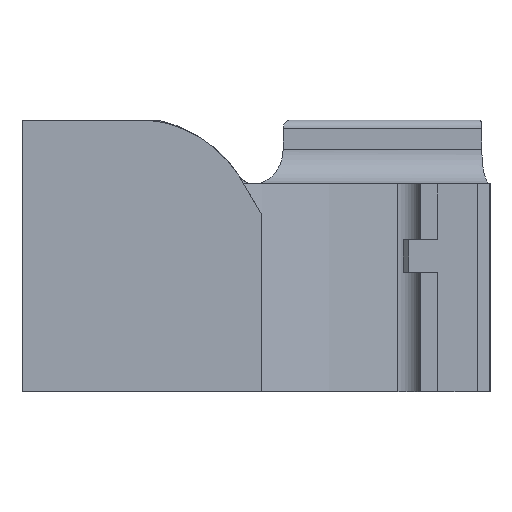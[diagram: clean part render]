
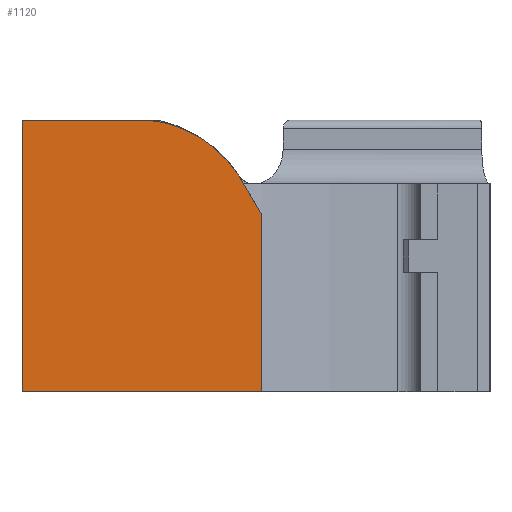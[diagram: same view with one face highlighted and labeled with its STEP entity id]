
A CAD part, front view. The second image highlights one B-rep face of the part: STEP entity #1120.
In plain terms, the highlighted planar face has unit normal (0, -1, 0).
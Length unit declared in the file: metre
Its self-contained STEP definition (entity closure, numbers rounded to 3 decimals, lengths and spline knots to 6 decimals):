
#39=PLANE('',#1247);
#86=FACE_OUTER_BOUND('',#145,.T.);
#145=EDGE_LOOP('',(#937,#938,#939,#940,#941,#942));
#189=LINE('',#1629,#303);
#198=LINE('',#1653,#312);
#215=LINE('',#1703,#329);
#235=LINE('',#1781,#349);
#240=LINE('',#1798,#354);
#303=VECTOR('',#1289,0.01);
#312=VECTOR('',#1310,0.01);
#329=VECTOR('',#1353,0.016179);
#349=VECTOR('',#1417,0.014606);
#354=VECTOR('',#1432,0.01);
#416=CIRCLE('',#1175,0.005582);
#457=VERTEX_POINT('',#1626);
#458=VERTEX_POINT('',#1628);
#460=VERTEX_POINT('',#1634);
#467=VERTEX_POINT('',#1652);
#487=VERTEX_POINT('',#1702);
#523=VERTEX_POINT('',#1779);
#568=EDGE_CURVE('',#458,#457,#189,.T.);
#572=EDGE_CURVE('',#457,#460,#416,.T.);
#580=EDGE_CURVE('',#467,#458,#198,.T.);
#605=EDGE_CURVE('',#487,#467,#215,.T.);
#645=EDGE_CURVE('',#523,#460,#235,.T.);
#652=EDGE_CURVE('',#523,#487,#240,.T.);
#937=ORIENTED_EDGE('',*,*,#652,.T.);
#938=ORIENTED_EDGE('',*,*,#605,.T.);
#939=ORIENTED_EDGE('',*,*,#580,.T.);
#940=ORIENTED_EDGE('',*,*,#568,.T.);
#941=ORIENTED_EDGE('',*,*,#572,.T.);
#942=ORIENTED_EDGE('',*,*,#645,.F.);
#1120=ADVANCED_FACE('',(#86),#39,.F.);
#1175=AXIS2_PLACEMENT_3D('',#1636,#1296,#1297);
#1247=AXIS2_PLACEMENT_3D('',#1922,#1526,#1527);
#1289=DIRECTION('',(-0.505,0.,0.863));
#1296=DIRECTION('center_axis',(0.,-1.,0.));
#1297=DIRECTION('ref_axis',(0.844,0.,0.536));
#1310=DIRECTION('',(0.,0.,1.));
#1353=DIRECTION('',(1.,0.,0.));
#1417=DIRECTION('',(1.,0.,0.));
#1432=DIRECTION('',(0.,0.,-1.));
#1526=DIRECTION('center_axis',(0.,1.,0.));
#1527=DIRECTION('ref_axis',(-1.,0.,0.));
#1626=CARTESIAN_POINT('',(0.014302,-0.00635,0.003058));
#1628=CARTESIAN_POINT('',(0.015312,-0.00635,0.00133));
#1629=CARTESIAN_POINT('',(0.014512,-0.00635,0.002699));
#1634=CARTESIAN_POINT('',(0.010128,-0.00635,0.00562));
#1636=CARTESIAN_POINT('Origin',(0.009592,-0.00635,0.000064));
#1652=CARTESIAN_POINT('',(0.015312,-0.00635,-0.006826));
#1653=CARTESIAN_POINT('',(0.015312,-0.00635,-0.006826));
#1702=CARTESIAN_POINT('',(0.004366,-0.00635,-0.006826));
#1703=CARTESIAN_POINT('',(-0.00605,-0.00635,-0.006826));
#1779=CARTESIAN_POINT('',(0.004366,-0.00635,0.00562));
#1781=CARTESIAN_POINT('',(-0.00605,-0.00635,0.00562));
#1798=CARTESIAN_POINT('',(0.004366,-0.00635,0.00562));
#1922=CARTESIAN_POINT('Origin',(-0.000603,-0.00635,0.00562));
